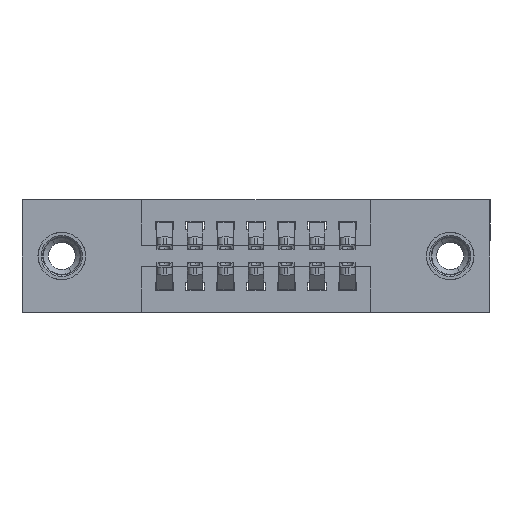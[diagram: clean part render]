
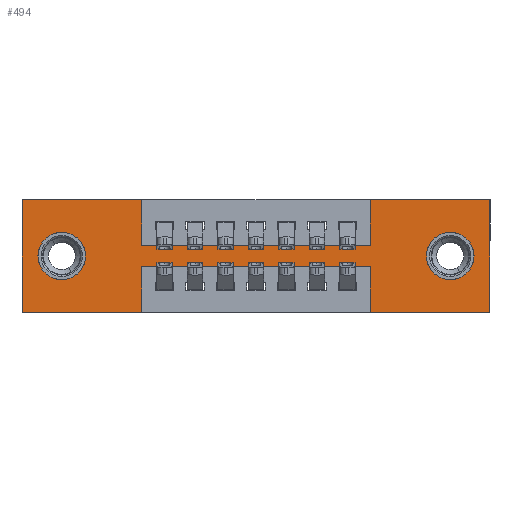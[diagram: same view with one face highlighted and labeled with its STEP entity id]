
A CAD part, front view. The second image highlights one B-rep face of the part: STEP entity #494.
In plain terms, the highlighted planar face has unit normal (0, -1, 0).
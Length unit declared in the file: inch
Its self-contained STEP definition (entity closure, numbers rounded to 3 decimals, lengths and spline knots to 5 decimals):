
#2 = LINE ( 'NONE', #5952, #9045 ) ;
#243 = EDGE_CURVE ( 'NONE', #13917, #1741, #3703, .T. ) ;
#494 = ADVANCED_FACE ( 'NONE', ( #12372, #10696, #7569 ), #13760, .T. ) ;
#565 = CARTESIAN_POINT ( 'NONE',  ( 1.405, 0., -0.185 ) ) ;
#699 = EDGE_LOOP ( 'NONE', ( #14388, #826, #4867, #761, #7258, #12747, #12679, #13168, #3061, #11526, #7544, #14765 ) ) ;
#740 = LINE ( 'NONE', #10340, #3526 ) ;
#761 = ORIENTED_EDGE ( 'NONE', *, *, #11060, .F. ) ;
#826 = ORIENTED_EDGE ( 'NONE', *, *, #4344, .F. ) ;
#898 = CARTESIAN_POINT ( 'NONE',  ( 1.405, 0., -0.185 ) ) ;
#943 = DIRECTION ( 'NONE',  ( 0., 0., -1. ) ) ;
#1073 = VECTOR ( 'NONE', #4203, 39.37008 ) ;
#1238 = DIRECTION ( 'NONE',  ( 0., 0., 1. ) ) ;
#1361 = CARTESIAN_POINT ( 'NONE',  ( 0.3925, 0., -0.22 ) ) ;
#1459 = AXIS2_PLACEMENT_3D ( 'NONE', #6450, #10153, #14694 ) ;
#1588 = LINE ( 'NONE', #3544, #13822 ) ;
#1741 = VERTEX_POINT ( 'NONE', #4236 ) ;
#1841 = DIRECTION ( 'NONE',  ( 0., 0., 1. ) ) ;
#1907 = DIRECTION ( 'NONE',  ( 0., 0., -1. ) ) ;
#2179 = LINE ( 'NONE', #13749, #15111 ) ;
#2250 = CARTESIAN_POINT ( 'NONE',  ( 0., 0., 0. ) ) ;
#2276 = VERTEX_POINT ( 'NONE', #9605 ) ;
#2280 = EDGE_LOOP ( 'NONE', ( #13409, #6380 ) ) ;
#2515 = VERTEX_POINT ( 'NONE', #6812 ) ;
#2545 = VECTOR ( 'NONE', #8052, 39.37008 ) ;
#2612 = EDGE_CURVE ( 'NONE', #3197, #2276, #1588, .T. ) ;
#2679 = AXIS2_PLACEMENT_3D ( 'NONE', #898, #3289, #943 ) ;
#2732 = EDGE_CURVE ( 'NONE', #2832, #5674, #5678, .T. ) ;
#2832 = VERTEX_POINT ( 'NONE', #11185 ) ;
#2848 = VERTEX_POINT ( 'NONE', #7631 ) ;
#3005 = VERTEX_POINT ( 'NONE', #3518 ) ;
#3061 = ORIENTED_EDGE ( 'NONE', *, *, #4083, .F. ) ;
#3128 = VECTOR ( 'NONE', #9713, 39.37008 ) ;
#3197 = VERTEX_POINT ( 'NONE', #6584 ) ;
#3289 = DIRECTION ( 'NONE',  ( 0., 1., 0. ) ) ;
#3308 = DIRECTION ( 'NONE',  ( 0., 0., 1. ) ) ;
#3350 = EDGE_CURVE ( 'NONE', #12357, #2832, #9689, .T. ) ;
#3357 = VERTEX_POINT ( 'NONE', #10169 ) ;
#3514 = LINE ( 'NONE', #5109, #3128 ) ;
#3518 = CARTESIAN_POINT ( 'NONE',  ( 1.405, 0., -0.107 ) ) ;
#3526 = VECTOR ( 'NONE', #8018, 39.37008 ) ;
#3544 = CARTESIAN_POINT ( 'NONE',  ( 0.3925, 0., -0.15 ) ) ;
#3703 = CIRCLE ( 'NONE', #1459, 0.078 ) ;
#3710 = CARTESIAN_POINT ( 'NONE',  ( 1.405, 0., -0.263 ) ) ;
#3830 = VECTOR ( 'NONE', #9277, 39.37008 ) ;
#4083 = EDGE_CURVE ( 'NONE', #5674, #3197, #9120, .T. ) ;
#4203 = DIRECTION ( 'NONE',  ( 0., 0., 1. ) ) ;
#4236 = CARTESIAN_POINT ( 'NONE',  ( 0.13, 0., -0.263 ) ) ;
#4344 = EDGE_CURVE ( 'NONE', #3357, #12143, #12479, .T. ) ;
#4399 = CARTESIAN_POINT ( 'NONE',  ( 0.13, 0., -0.107 ) ) ;
#4477 = CARTESIAN_POINT ( 'NONE',  ( 0.3925, 0., -0.22 ) ) ;
#4626 = DIRECTION ( 'NONE',  ( -1., 0., 0. ) ) ;
#4867 = ORIENTED_EDGE ( 'NONE', *, *, #11472, .F. ) ;
#5109 = CARTESIAN_POINT ( 'NONE',  ( 0., 0., -0.37 ) ) ;
#5586 = DIRECTION ( 'NONE',  ( 0., 0., -1. ) ) ;
#5663 = VECTOR ( 'NONE', #3308, 39.37008 ) ;
#5674 = VERTEX_POINT ( 'NONE', #10298 ) ;
#5678 = LINE ( 'NONE', #2250, #3830 ) ;
#5880 = CARTESIAN_POINT ( 'NONE',  ( 0.13, 0., -0.185 ) ) ;
#5916 = LINE ( 'NONE', #12934, #2545 ) ;
#5952 = CARTESIAN_POINT ( 'NONE',  ( 0.3925, 0., -0.37 ) ) ;
#6012 = VERTEX_POINT ( 'NONE', #6085 ) ;
#6085 = CARTESIAN_POINT ( 'NONE',  ( 1.1425, 0., 0. ) ) ;
#6380 = ORIENTED_EDGE ( 'NONE', *, *, #10648, .T. ) ;
#6450 = CARTESIAN_POINT ( 'NONE',  ( 0.13, 0., -0.185 ) ) ;
#6479 = EDGE_CURVE ( 'NONE', #12143, #2515, #2, .T. ) ;
#6584 = CARTESIAN_POINT ( 'NONE',  ( 0.3925, 0., -0.15 ) ) ;
#6812 = CARTESIAN_POINT ( 'NONE',  ( 0.3925, 0., -0.37 ) ) ;
#6846 = EDGE_CURVE ( 'NONE', #2515, #12357, #3514, .T. ) ;
#7067 = DIRECTION ( 'NONE',  ( 0., 1., 0. ) ) ;
#7258 = ORIENTED_EDGE ( 'NONE', *, *, #8028, .F. ) ;
#7302 = VECTOR ( 'NONE', #4626, 39.37008 ) ;
#7544 = ORIENTED_EDGE ( 'NONE', *, *, #3350, .F. ) ;
#7569 = FACE_OUTER_BOUND ( 'NONE', #699, .T. ) ;
#7619 = EDGE_CURVE ( 'NONE', #3005, #10082, #9033, .T. ) ;
#7631 = CARTESIAN_POINT ( 'NONE',  ( 1.535, 0., 0. ) ) ;
#7663 = DIRECTION ( 'NONE',  ( 0., -1., 0. ) ) ;
#8018 = DIRECTION ( 'NONE',  ( -1., 0., 0. ) ) ;
#8028 = EDGE_CURVE ( 'NONE', #2848, #13122, #12184, .T. ) ;
#8052 = DIRECTION ( 'NONE',  ( 1., 0., 0. ) ) ;
#8760 = DIRECTION ( 'NONE',  ( 0., 0., -1. ) ) ;
#9033 = CIRCLE ( 'NONE', #12366, 0.078 ) ;
#9045 = VECTOR ( 'NONE', #15217, 39.37008 ) ;
#9120 = LINE ( 'NONE', #12094, #13786 ) ;
#9277 = DIRECTION ( 'NONE',  ( 1., 0., 0. ) ) ;
#9491 = ORIENTED_EDGE ( 'NONE', *, *, #7619, .T. ) ;
#9605 = CARTESIAN_POINT ( 'NONE',  ( 1.1425, 0., -0.15 ) ) ;
#9689 = LINE ( 'NONE', #10379, #5663 ) ;
#9713 = DIRECTION ( 'NONE',  ( -1., 0., 0. ) ) ;
#9860 = EDGE_LOOP ( 'NONE', ( #9491, #10127 ) ) ;
#10082 = VERTEX_POINT ( 'NONE', #3710 ) ;
#10127 = ORIENTED_EDGE ( 'NONE', *, *, #13980, .T. ) ;
#10153 = DIRECTION ( 'NONE',  ( 0., 1., 0. ) ) ;
#10169 = CARTESIAN_POINT ( 'NONE',  ( 1.1425, 0., -0.22 ) ) ;
#10298 = CARTESIAN_POINT ( 'NONE',  ( 0.3925, 0., 0. ) ) ;
#10327 = CIRCLE ( 'NONE', #2679, 0.078 ) ;
#10340 = CARTESIAN_POINT ( 'NONE',  ( 0., 0., -0.37 ) ) ;
#10379 = CARTESIAN_POINT ( 'NONE',  ( 0., 0., 0. ) ) ;
#10479 = VERTEX_POINT ( 'NONE', #14032 ) ;
#10648 = EDGE_CURVE ( 'NONE', #1741, #13917, #14248, .T. ) ;
#10696 = FACE_BOUND ( 'NONE', #2280, .T. ) ;
#10720 = LINE ( 'NONE', #14705, #1073 ) ;
#11060 = EDGE_CURVE ( 'NONE', #13122, #10479, #740, .T. ) ;
#11175 = CARTESIAN_POINT ( 'NONE',  ( 1.535, 0., 0. ) ) ;
#11185 = CARTESIAN_POINT ( 'NONE',  ( 0., 0., 0. ) ) ;
#11472 = EDGE_CURVE ( 'NONE', #10479, #3357, #10720, .T. ) ;
#11526 = ORIENTED_EDGE ( 'NONE', *, *, #2732, .F. ) ;
#12043 = EDGE_CURVE ( 'NONE', #6012, #2848, #5916, .T. ) ;
#12094 = CARTESIAN_POINT ( 'NONE',  ( 0.3925, 0., 0. ) ) ;
#12143 = VERTEX_POINT ( 'NONE', #1361 ) ;
#12184 = LINE ( 'NONE', #11175, #14925 ) ;
#12326 = CARTESIAN_POINT ( 'NONE',  ( 1.535, 0., -0.37 ) ) ;
#12357 = VERTEX_POINT ( 'NONE', #14542 ) ;
#12366 = AXIS2_PLACEMENT_3D ( 'NONE', #565, #14807, #1907 ) ;
#12372 = FACE_BOUND ( 'NONE', #9860, .T. ) ;
#12479 = LINE ( 'NONE', #4477, #7302 ) ;
#12590 = AXIS2_PLACEMENT_3D ( 'NONE', #5880, #7067, #1238 ) ;
#12679 = ORIENTED_EDGE ( 'NONE', *, *, #13874, .F. ) ;
#12747 = ORIENTED_EDGE ( 'NONE', *, *, #12043, .F. ) ;
#12882 = AXIS2_PLACEMENT_3D ( 'NONE', #14898, #7663, #5586 ) ;
#12934 = CARTESIAN_POINT ( 'NONE',  ( 0., 0., 0. ) ) ;
#12955 = DIRECTION ( 'NONE',  ( 1., 0., 0. ) ) ;
#13122 = VERTEX_POINT ( 'NONE', #12326 ) ;
#13168 = ORIENTED_EDGE ( 'NONE', *, *, #2612, .F. ) ;
#13186 = DIRECTION ( 'NONE',  ( 0., 0., -1. ) ) ;
#13409 = ORIENTED_EDGE ( 'NONE', *, *, #243, .T. ) ;
#13749 = CARTESIAN_POINT ( 'NONE',  ( 1.1425, 0., 0. ) ) ;
#13760 = PLANE ( 'NONE',  #12882 ) ;
#13786 = VECTOR ( 'NONE', #13186, 39.37008 ) ;
#13822 = VECTOR ( 'NONE', #12955, 39.37008 ) ;
#13874 = EDGE_CURVE ( 'NONE', #2276, #6012, #2179, .T. ) ;
#13917 = VERTEX_POINT ( 'NONE', #4399 ) ;
#13980 = EDGE_CURVE ( 'NONE', #10082, #3005, #10327, .T. ) ;
#14032 = CARTESIAN_POINT ( 'NONE',  ( 1.1425, 0., -0.37 ) ) ;
#14248 = CIRCLE ( 'NONE', #12590, 0.078 ) ;
#14388 = ORIENTED_EDGE ( 'NONE', *, *, #6479, .F. ) ;
#14542 = CARTESIAN_POINT ( 'NONE',  ( 0., 0., -0.37 ) ) ;
#14694 = DIRECTION ( 'NONE',  ( 0., 0., 1. ) ) ;
#14705 = CARTESIAN_POINT ( 'NONE',  ( 1.1425, 0., -0.37 ) ) ;
#14765 = ORIENTED_EDGE ( 'NONE', *, *, #6846, .F. ) ;
#14807 = DIRECTION ( 'NONE',  ( 0., 1., 0. ) ) ;
#14898 = CARTESIAN_POINT ( 'NONE',  ( 0., 0., -0.37 ) ) ;
#14925 = VECTOR ( 'NONE', #8760, 39.37008 ) ;
#15111 = VECTOR ( 'NONE', #1841, 39.37008 ) ;
#15217 = DIRECTION ( 'NONE',  ( 0., 0., -1. ) ) ;
